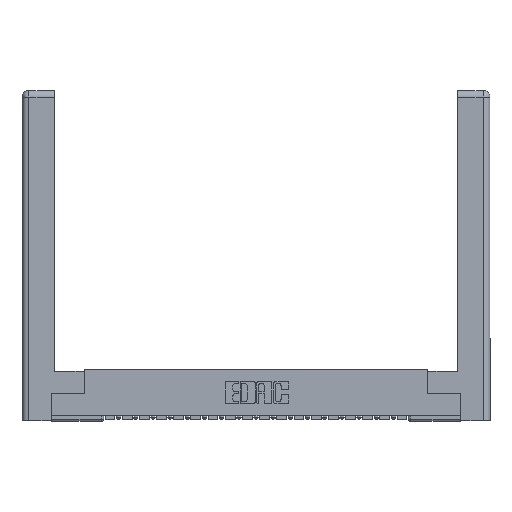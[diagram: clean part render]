
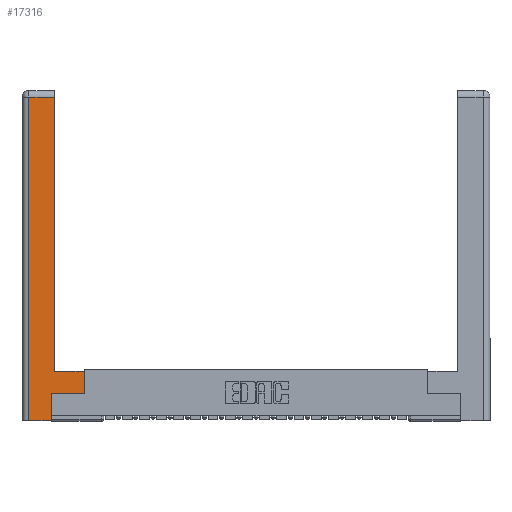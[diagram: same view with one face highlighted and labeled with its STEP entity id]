
A CAD part, top view. The second image highlights one B-rep face of the part: STEP entity #17316.
In plain terms, the highlighted planar face has unit normal (0, 0, 1).
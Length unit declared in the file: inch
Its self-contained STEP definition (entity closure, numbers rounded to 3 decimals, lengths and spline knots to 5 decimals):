
#245 = EDGE_CURVE ( 'NONE', #18246, #11229, #11751, .T. ) ;
#287 = LINE ( 'NONE', #13945, #6654 ) ;
#351 = LINE ( 'NONE', #18412, #8828 ) ;
#404 = CARTESIAN_POINT ( 'NONE',  ( 0.295, 0.45, 0. ) ) ;
#856 = DIRECTION ( 'NONE',  ( 1., 0., 0. ) ) ;
#1026 = CARTESIAN_POINT ( 'NONE',  ( 0., 0., 0. ) ) ;
#1344 = VECTOR ( 'NONE', #8985, 39.37008 ) ;
#1439 = EDGE_CURVE ( 'NONE', #9015, #15199, #21766, .T. ) ;
#2402 = VECTOR ( 'NONE', #5025, 39.37008 ) ;
#2702 = ORIENTED_EDGE ( 'NONE', *, *, #245, .T. ) ;
#3327 = VERTEX_POINT ( 'NONE', #15813 ) ;
#3490 = FACE_OUTER_BOUND ( 'NONE', #13883, .T. ) ;
#3953 = DIRECTION ( 'NONE',  ( 0., 1., 0. ) ) ;
#4132 = ORIENTED_EDGE ( 'NONE', *, *, #1439, .T. ) ;
#4577 = DIRECTION ( 'NONE',  ( 1., 0., 0. ) ) ;
#4588 = DIRECTION ( 'NONE',  ( -1., 0., 0. ) ) ;
#5025 = DIRECTION ( 'NONE',  ( 0., 1., 0. ) ) ;
#5107 = CARTESIAN_POINT ( 'NONE',  ( 0.295, 0.45, 0. ) ) ;
#6517 = CARTESIAN_POINT ( 'NONE',  ( 0.265, 0.245, 0. ) ) ;
#6638 = ORIENTED_EDGE ( 'NONE', *, *, #18355, .T. ) ;
#6654 = VECTOR ( 'NONE', #8813, 39.37008 ) ;
#7083 = VERTEX_POINT ( 'NONE', #20769 ) ;
#7187 = VECTOR ( 'NONE', #13309, 39.37008 ) ;
#7474 = VECTOR ( 'NONE', #856, 39.37008 ) ;
#7935 = CARTESIAN_POINT ( 'NONE',  ( 0.265, 0.245, 0. ) ) ;
#7989 = PLANE ( 'NONE',  #21731 ) ;
#8564 = DIRECTION ( 'NONE',  ( 0., -1., 0. ) ) ;
#8813 = DIRECTION ( 'NONE',  ( 0., 1., 0. ) ) ;
#8828 = VECTOR ( 'NONE', #8564, 39.37008 ) ;
#8985 = DIRECTION ( 'NONE',  ( -1., 0., 0. ) ) ;
#9015 = VERTEX_POINT ( 'NONE', #20839 ) ;
#9575 = VERTEX_POINT ( 'NONE', #12743 ) ;
#9615 = ORIENTED_EDGE ( 'NONE', *, *, #10290, .T. ) ;
#10290 = EDGE_CURVE ( 'NONE', #3327, #9575, #17537, .T. ) ;
#10624 = EDGE_CURVE ( 'NONE', #11714, #7083, #20957, .T. ) ;
#11229 = VERTEX_POINT ( 'NONE', #13359 ) ;
#11690 = CARTESIAN_POINT ( 'NONE',  ( 0.565, 0.45, 0. ) ) ;
#11714 = VERTEX_POINT ( 'NONE', #18133 ) ;
#11751 = LINE ( 'NONE', #21544, #16264 ) ;
#12050 = LINE ( 'NONE', #11690, #16294 ) ;
#12743 = CARTESIAN_POINT ( 'NONE',  ( 0.265, 0., 0. ) ) ;
#13122 = DIRECTION ( 'NONE',  ( 0., 0., -1. ) ) ;
#13309 = DIRECTION ( 'NONE',  ( -1., 0., 0. ) ) ;
#13359 = CARTESIAN_POINT ( 'NONE',  ( 0.565, 0.245, 0. ) ) ;
#13883 = EDGE_LOOP ( 'NONE', ( #18078, #15763, #21826, #9615, #6638, #2702, #16827, #4132 ) ) ;
#13945 = CARTESIAN_POINT ( 'NONE',  ( 0.295, 3., 0. ) ) ;
#15000 = EDGE_CURVE ( 'NONE', #7083, #3327, #351, .T. ) ;
#15070 = EDGE_CURVE ( 'NONE', #11229, #9015, #12050, .T. ) ;
#15199 = VERTEX_POINT ( 'NONE', #5107 ) ;
#15763 = ORIENTED_EDGE ( 'NONE', *, *, #10624, .T. ) ;
#15813 = CARTESIAN_POINT ( 'NONE',  ( 0.0615, 0., 0. ) ) ;
#15908 = LINE ( 'NONE', #6517, #2402 ) ;
#16196 = CARTESIAN_POINT ( 'NONE',  ( 0.265, 0., 0. ) ) ;
#16264 = VECTOR ( 'NONE', #4577, 39.37008 ) ;
#16294 = VECTOR ( 'NONE', #3953, 39.37008 ) ;
#16827 = ORIENTED_EDGE ( 'NONE', *, *, #15070, .T. ) ;
#16966 = EDGE_CURVE ( 'NONE', #15199, #11714, #287, .T. ) ;
#17316 = ADVANCED_FACE ( 'NONE', ( #3490 ), #7989, .F. ) ;
#17537 = LINE ( 'NONE', #16196, #7474 ) ;
#18078 = ORIENTED_EDGE ( 'NONE', *, *, #16966, .T. ) ;
#18133 = CARTESIAN_POINT ( 'NONE',  ( 0.295, 2.94, 0. ) ) ;
#18246 = VERTEX_POINT ( 'NONE', #7935 ) ;
#18355 = EDGE_CURVE ( 'NONE', #9575, #18246, #15908, .T. ) ;
#18412 = CARTESIAN_POINT ( 'NONE',  ( 0.0615, 0., 0. ) ) ;
#20769 = CARTESIAN_POINT ( 'NONE',  ( 0.0615, 2.94, 0. ) ) ;
#20839 = CARTESIAN_POINT ( 'NONE',  ( 0.565, 0.45, 0. ) ) ;
#20957 = LINE ( 'NONE', #21973, #7187 ) ;
#21544 = CARTESIAN_POINT ( 'NONE',  ( 0.565, 0.245, 0. ) ) ;
#21731 = AXIS2_PLACEMENT_3D ( 'NONE', #1026, #13122, #4588 ) ;
#21766 = LINE ( 'NONE', #404, #1344 ) ;
#21826 = ORIENTED_EDGE ( 'NONE', *, *, #15000, .T. ) ;
#21973 = CARTESIAN_POINT ( 'NONE',  ( 0.0615, 2.94, 0. ) ) ;
